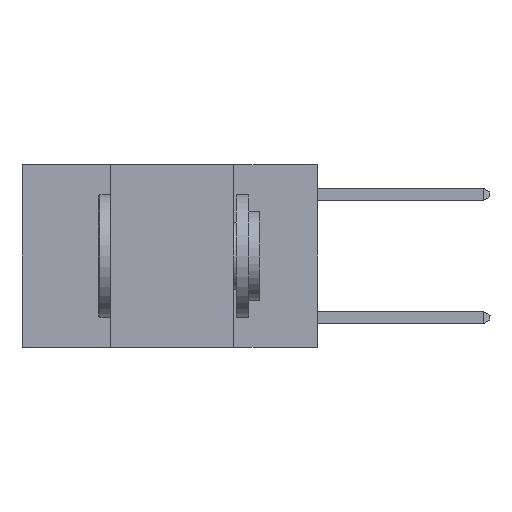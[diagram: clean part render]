
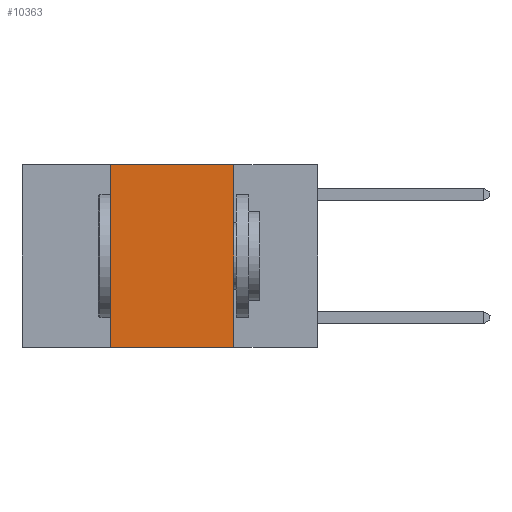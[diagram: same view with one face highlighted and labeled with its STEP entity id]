
A CAD part, left-side view. The second image highlights one B-rep face of the part: STEP entity #10363.
In plain terms, the highlighted planar face has unit normal (-1, 0, 0).
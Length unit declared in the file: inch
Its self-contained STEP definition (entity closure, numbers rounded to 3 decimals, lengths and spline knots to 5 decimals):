
#768 = EDGE_LOOP ( 'NONE', ( #6400, #11030, #7859, #16112 ) ) ;
#958 = DIRECTION ( 'NONE',  ( 0., 0., -1. ) ) ;
#1598 = VECTOR ( 'NONE', #16790, 39.37008 ) ;
#1817 = DIRECTION ( 'NONE',  ( 0., -1., 0. ) ) ;
#2482 = VECTOR ( 'NONE', #1817, 39.37008 ) ;
#3572 = DIRECTION ( 'NONE',  ( 0., 0., -1. ) ) ;
#3719 = VERTEX_POINT ( 'NONE', #15886 ) ;
#3764 = VECTOR ( 'NONE', #3572, 39.37008 ) ;
#4066 = DIRECTION ( 'NONE',  ( 0., -1., 0. ) ) ;
#5119 = CARTESIAN_POINT ( 'NONE',  ( 0., 0.17, 0. ) ) ;
#5195 = LINE ( 'NONE', #5119, #3764 ) ;
#5448 = FACE_OUTER_BOUND ( 'NONE', #768, .T. ) ;
#6100 = LINE ( 'NONE', #9548, #2482 ) ;
#6400 = ORIENTED_EDGE ( 'NONE', *, *, #14814, .F. ) ;
#7121 = PLANE ( 'NONE',  #10948 ) ;
#7859 = ORIENTED_EDGE ( 'NONE', *, *, #13810, .F. ) ;
#8205 = CARTESIAN_POINT ( 'NONE',  ( 0., 0.42, 0. ) ) ;
#8717 = VERTEX_POINT ( 'NONE', #13049 ) ;
#9548 = CARTESIAN_POINT ( 'NONE',  ( 0., 0.6, -0.37 ) ) ;
#10267 = DIRECTION ( 'NONE',  ( 1., 0., 0. ) ) ;
#10363 = ADVANCED_FACE ( 'NONE', ( #5448 ), #7121, .F. ) ;
#10947 = EDGE_CURVE ( 'NONE', #13414, #8717, #15353, .T. ) ;
#10948 = AXIS2_PLACEMENT_3D ( 'NONE', #19395, #10267, #958 ) ;
#11030 = ORIENTED_EDGE ( 'NONE', *, *, #10947, .F. ) ;
#11081 = VERTEX_POINT ( 'NONE', #15160 ) ;
#12751 = EDGE_CURVE ( 'NONE', #11081, #3719, #6100, .T. ) ;
#13049 = CARTESIAN_POINT ( 'NONE',  ( 0., 0.17, 0. ) ) ;
#13414 = VERTEX_POINT ( 'NONE', #8205 ) ;
#13810 = EDGE_CURVE ( 'NONE', #11081, #13414, #13984, .T. ) ;
#13984 = LINE ( 'NONE', #15244, #1598 ) ;
#14814 = EDGE_CURVE ( 'NONE', #8717, #3719, #5195, .T. ) ;
#15160 = CARTESIAN_POINT ( 'NONE',  ( 0., 0.42, -0.37 ) ) ;
#15244 = CARTESIAN_POINT ( 'NONE',  ( 0., 0.42, 0. ) ) ;
#15353 = LINE ( 'NONE', #19434, #18874 ) ;
#15886 = CARTESIAN_POINT ( 'NONE',  ( 0., 0.17, -0.37 ) ) ;
#16112 = ORIENTED_EDGE ( 'NONE', *, *, #12751, .T. ) ;
#16790 = DIRECTION ( 'NONE',  ( 0., 0., 1. ) ) ;
#18874 = VECTOR ( 'NONE', #4066, 39.37008 ) ;
#19395 = CARTESIAN_POINT ( 'NONE',  ( 0., 0.6, 0. ) ) ;
#19434 = CARTESIAN_POINT ( 'NONE',  ( 0., 0.6, 0. ) ) ;
